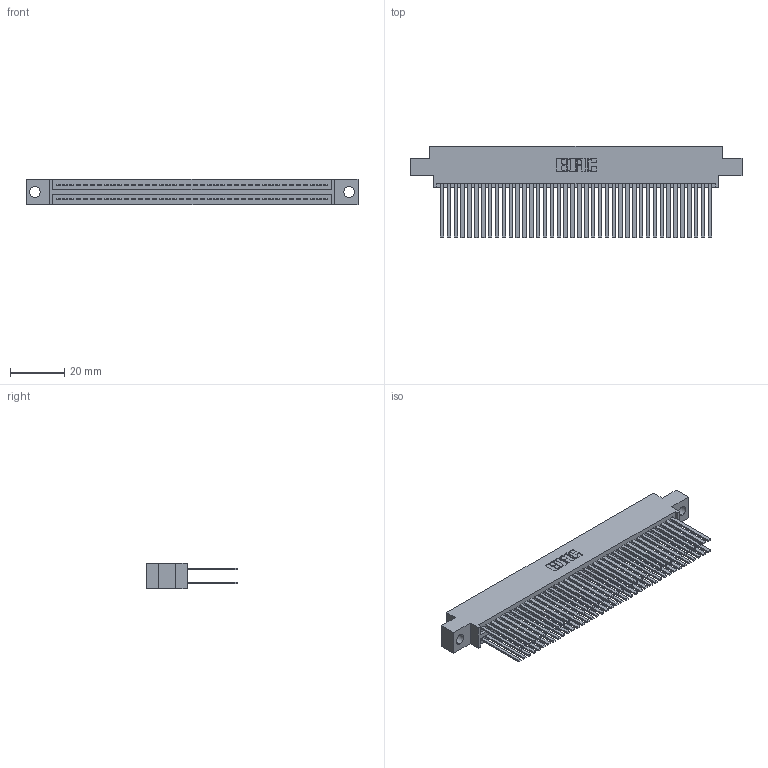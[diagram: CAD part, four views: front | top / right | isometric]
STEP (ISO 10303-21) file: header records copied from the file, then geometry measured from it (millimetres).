
FILE_DESCRIPTION (( 'STEP AP203' ), '1' );
FILE_NAME ('345-080-544-804.STEP', '2018-10-03T18:36:48', ( '' ), ( '' ), 'SwSTEP 2.0', 'SolidWorks 2016', '' );
FILE_SCHEMA (( 'CONFIG_CONTROL_DESIGN' ));
Length unit declared in the file: inch
Products named in the file (3): 345-292-001_345-293-144; 345 Part_0.170 Offset - 0.156 Dia-TH; 345-080-544-804
Assembly tree (81 placements, depth 2):
  345-080-544-804
    345 Part_0.170 Offset - 0.156 Dia-TH
    345-292-001_345-293-144  x80
Bounding box: 122.81 x 33.96 x 9.4 mm (x, y, z)
Volume: 12831.4 mm3; surface area: 22173.8 mm2
Topology: 81 solids, 81 shells, 3650 faces, 10833 edges, 7114 vertices
Faces by surface type: plane 2404, cylinder 1246
Entity records: 31605 total; most frequent: CARTESIAN_POINT 5300, ORIENTED_EDGE 5234, DIRECTION 4673, EDGE_CURVE 2617, LINE 2329, VECTOR 2329, VERTEX_POINT 1742, AXIS2_PLACEMENT_3D 1172
